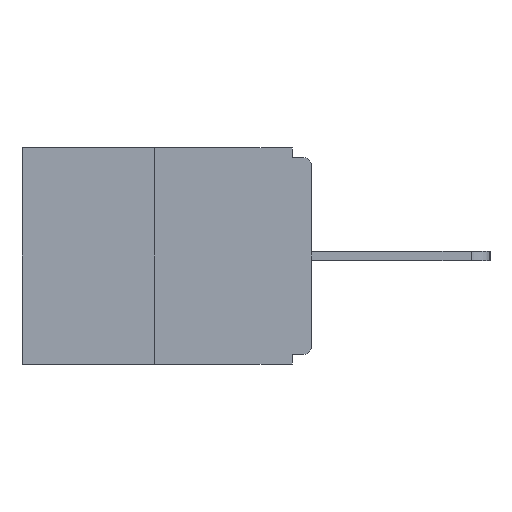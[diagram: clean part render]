
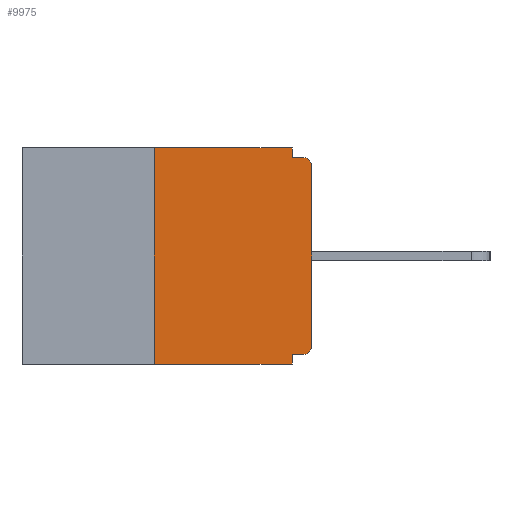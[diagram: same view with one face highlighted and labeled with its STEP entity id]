
A CAD part, left-side view. The second image highlights one B-rep face of the part: STEP entity #9975.
In plain terms, the highlighted planar face has unit normal (-1, 0, 0).
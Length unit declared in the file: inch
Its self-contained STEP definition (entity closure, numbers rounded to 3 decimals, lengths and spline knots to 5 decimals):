
#208 = DIRECTION ( 'NONE',  ( 0., 0., -1. ) ) ;
#300 = EDGE_CURVE ( 'NONE', #12429, #8597, #8773, .T. ) ;
#496 = EDGE_CURVE ( 'NONE', #11079, #12423, #9257, .T. ) ;
#517 = EDGE_CURVE ( 'NONE', #11898, #8597, #14602, .T. ) ;
#553 = LINE ( 'NONE', #13520, #966 ) ;
#733 = CARTESIAN_POINT ( 'NONE',  ( 0., 0., -0.03 ) ) ;
#824 = CARTESIAN_POINT ( 'NONE',  ( 0., 0.46, -0.343 ) ) ;
#966 = VECTOR ( 'NONE', #13455, 39.37008 ) ;
#1157 = ORIENTED_EDGE ( 'NONE', *, *, #10940, .F. ) ;
#1175 = LINE ( 'NONE', #12075, #13317 ) ;
#1185 = DIRECTION ( 'NONE',  ( 0., 0., -1. ) ) ;
#1199 = PLANE ( 'NONE',  #10982 ) ;
#1311 = CARTESIAN_POINT ( 'NONE',  ( 0., 0.015, -0.328 ) ) ;
#1416 = VECTOR ( 'NONE', #208, 39.37008 ) ;
#2177 = VERTEX_POINT ( 'NONE', #7261 ) ;
#2459 = DIRECTION ( 'NONE',  ( 0., 0., -1. ) ) ;
#3009 = DIRECTION ( 'NONE',  ( 0., -1., 0. ) ) ;
#3043 = CARTESIAN_POINT ( 'NONE',  ( 0., 0., -0.328 ) ) ;
#3217 = DIRECTION ( 'NONE',  ( 0., -1., 0. ) ) ;
#3299 = VERTEX_POINT ( 'NONE', #3928 ) ;
#3543 = FACE_OUTER_BOUND ( 'NONE', #8454, .T. ) ;
#3747 = DIRECTION ( 'NONE',  ( 0., -1., 0. ) ) ;
#3928 = CARTESIAN_POINT ( 'NONE',  ( 0., 0., -0.313 ) ) ;
#4314 = LINE ( 'NONE', #3043, #12874 ) ;
#4399 = ORIENTED_EDGE ( 'NONE', *, *, #9133, .F. ) ;
#4554 = VERTEX_POINT ( 'NONE', #13182 ) ;
#4618 = EDGE_CURVE ( 'NONE', #11079, #4554, #1175, .T. ) ;
#4647 = LINE ( 'NONE', #7459, #1416 ) ;
#4770 = ORIENTED_EDGE ( 'NONE', *, *, #300, .T. ) ;
#4809 = CARTESIAN_POINT ( 'NONE',  ( 0., 0.46, 0. ) ) ;
#4883 = CARTESIAN_POINT ( 'NONE',  ( 0., 0.46, 0. ) ) ;
#4914 = EDGE_CURVE ( 'NONE', #2177, #11898, #553, .T. ) ;
#5313 = CARTESIAN_POINT ( 'NONE',  ( 0., 0., -0.015 ) ) ;
#5529 = CARTESIAN_POINT ( 'NONE',  ( 0., 0.015, -0.015 ) ) ;
#5533 = CARTESIAN_POINT ( 'NONE',  ( 0., 0.031, -0.343 ) ) ;
#6115 = EDGE_CURVE ( 'NONE', #3299, #12429, #9948, .T. ) ;
#7147 = ORIENTED_EDGE ( 'NONE', *, *, #4618, .F. ) ;
#7261 = CARTESIAN_POINT ( 'NONE',  ( 0., 0.031, 0. ) ) ;
#7459 = CARTESIAN_POINT ( 'NONE',  ( 0., 0.031, -0.343 ) ) ;
#8338 = DIRECTION ( 'NONE',  ( -1., 0., 0. ) ) ;
#8454 = EDGE_LOOP ( 'NONE', ( #12611, #7147, #10114, #1157, #4399, #10431, #13298, #4770, #10767, #13645 ) ) ;
#8495 = VERTEX_POINT ( 'NONE', #11977 ) ;
#8597 = VERTEX_POINT ( 'NONE', #5529 ) ;
#8773 = CIRCLE ( 'NONE', #12872, 0.015 ) ;
#9133 = EDGE_CURVE ( 'NONE', #10025, #8495, #4314, .T. ) ;
#9218 = CARTESIAN_POINT ( 'NONE',  ( 0., 0.031, -0.015 ) ) ;
#9257 = LINE ( 'NONE', #824, #9914 ) ;
#9433 = DIRECTION ( 'NONE',  ( 1., 0., 0. ) ) ;
#9914 = VECTOR ( 'NONE', #3217, 39.37008 ) ;
#9926 = CARTESIAN_POINT ( 'NONE',  ( 0., 0.25, -0.343 ) ) ;
#9948 = LINE ( 'NONE', #11713, #12780 ) ;
#9975 = ADVANCED_FACE ( 'NONE', ( #3543 ), #1199, .F. ) ;
#10025 = VERTEX_POINT ( 'NONE', #1311 ) ;
#10063 = LINE ( 'NONE', #4883, #12223 ) ;
#10114 = ORIENTED_EDGE ( 'NONE', *, *, #496, .T. ) ;
#10431 = ORIENTED_EDGE ( 'NONE', *, *, #10774, .T. ) ;
#10767 = ORIENTED_EDGE ( 'NONE', *, *, #517, .F. ) ;
#10774 = EDGE_CURVE ( 'NONE', #10025, #3299, #13010, .T. ) ;
#10848 = DIRECTION ( 'NONE',  ( 0., 0., -1. ) ) ;
#10907 = AXIS2_PLACEMENT_3D ( 'NONE', #14741, #8338, #1185 ) ;
#10940 = EDGE_CURVE ( 'NONE', #8495, #12423, #4647, .T. ) ;
#10982 = AXIS2_PLACEMENT_3D ( 'NONE', #4809, #9433, #2459 ) ;
#11079 = VERTEX_POINT ( 'NONE', #9926 ) ;
#11713 = CARTESIAN_POINT ( 'NONE',  ( 0., 0., 0. ) ) ;
#11745 = VECTOR ( 'NONE', #3009, 39.37008 ) ;
#11898 = VERTEX_POINT ( 'NONE', #9218 ) ;
#11977 = CARTESIAN_POINT ( 'NONE',  ( 0., 0.031, -0.328 ) ) ;
#11999 = DIRECTION ( 'NONE',  ( 0., 0., 1. ) ) ;
#12008 = DIRECTION ( 'NONE',  ( 0., 1., 0. ) ) ;
#12075 = CARTESIAN_POINT ( 'NONE',  ( 0., 0.25, 0. ) ) ;
#12223 = VECTOR ( 'NONE', #3747, 39.37008 ) ;
#12423 = VERTEX_POINT ( 'NONE', #5533 ) ;
#12429 = VERTEX_POINT ( 'NONE', #733 ) ;
#12611 = ORIENTED_EDGE ( 'NONE', *, *, #13150, .F. ) ;
#12780 = VECTOR ( 'NONE', #11999, 39.37008 ) ;
#12872 = AXIS2_PLACEMENT_3D ( 'NONE', #13693, #13743, #10848 ) ;
#12874 = VECTOR ( 'NONE', #12008, 39.37008 ) ;
#13010 = CIRCLE ( 'NONE', #10907, 0.015 ) ;
#13150 = EDGE_CURVE ( 'NONE', #4554, #2177, #10063, .T. ) ;
#13182 = CARTESIAN_POINT ( 'NONE',  ( 0., 0.25, 0. ) ) ;
#13298 = ORIENTED_EDGE ( 'NONE', *, *, #6115, .T. ) ;
#13317 = VECTOR ( 'NONE', #13435, 39.37008 ) ;
#13435 = DIRECTION ( 'NONE',  ( 0., 0., 1. ) ) ;
#13455 = DIRECTION ( 'NONE',  ( 0., 0., -1. ) ) ;
#13520 = CARTESIAN_POINT ( 'NONE',  ( 0., 0.031, 0. ) ) ;
#13645 = ORIENTED_EDGE ( 'NONE', *, *, #4914, .F. ) ;
#13693 = CARTESIAN_POINT ( 'NONE',  ( 0., 0.015, -0.03 ) ) ;
#13743 = DIRECTION ( 'NONE',  ( -1., 0., 0. ) ) ;
#14602 = LINE ( 'NONE', #5313, #11745 ) ;
#14741 = CARTESIAN_POINT ( 'NONE',  ( 0., 0.015, -0.313 ) ) ;
